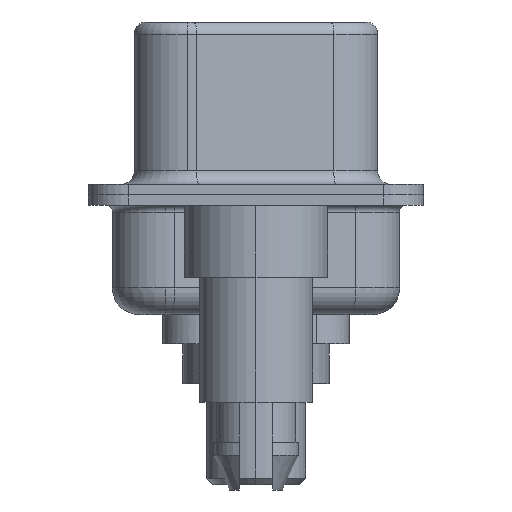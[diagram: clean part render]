
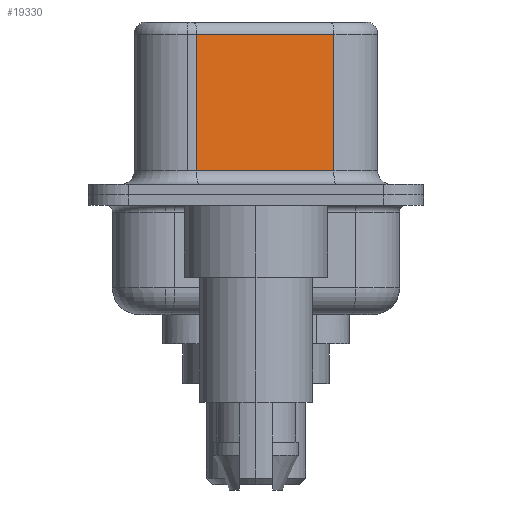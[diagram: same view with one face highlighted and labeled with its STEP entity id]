
A CAD part, left-side view. The second image highlights one B-rep face of the part: STEP entity #19330.
In plain terms, the highlighted planar face has unit normal (-0.985, -0.174, 0).
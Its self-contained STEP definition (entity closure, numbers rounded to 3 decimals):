
#17 = CARTESIAN_POINT ( 'NONE',  ( 4.585, -2.927, 6.52 ) ) ;
#502 = ORIENTED_EDGE ( 'NONE', *, *, #4506, .T. ) ;
#1041 = DIRECTION ( 'NONE',  ( -0.174, 0.985, 0. ) ) ;
#1089 = LINE ( 'NONE', #17, #16523 ) ;
#1209 = LINE ( 'NONE', #10187, #16655 ) ;
#1450 = DIRECTION ( 'NONE',  ( 0.174, -0.985, 0. ) ) ;
#4052 = EDGE_CURVE ( 'NONE', #6802, #17455, #1089, .T. ) ;
#4506 = EDGE_CURVE ( 'NONE', #6802, #15293, #11897, .T. ) ;
#5594 = CARTESIAN_POINT ( 'NONE',  ( 4.585, -2.927, 6.52 ) ) ;
#5728 = ORIENTED_EDGE ( 'NONE', *, *, #4052, .F. ) ;
#5755 = CARTESIAN_POINT ( 'NONE',  ( 3.675, 2.233, 6.02 ) ) ;
#6802 = VERTEX_POINT ( 'NONE', #10339 ) ;
#7949 = EDGE_CURVE ( 'NONE', #15293, #10622, #1209, .T. ) ;
#8872 = ORIENTED_EDGE ( 'NONE', *, *, #7949, .T. ) ;
#9713 = CARTESIAN_POINT ( 'NONE',  ( 3.675, 2.233, 0.9 ) ) ;
#10095 = DIRECTION ( 'NONE',  ( 0.985, 0.174, 0. ) ) ;
#10187 = CARTESIAN_POINT ( 'NONE',  ( 3.675, 2.233, 6.52 ) ) ;
#10339 = CARTESIAN_POINT ( 'NONE',  ( 4.585, -2.927, 6.02 ) ) ;
#10622 = VERTEX_POINT ( 'NONE', #9713 ) ;
#10651 = ORIENTED_EDGE ( 'NONE', *, *, #15370, .T. ) ;
#11198 = AXIS2_PLACEMENT_3D ( 'NONE', #5594, #10095, #1041 ) ;
#11897 = LINE ( 'NONE', #12663, #15821 ) ;
#11906 = CARTESIAN_POINT ( 'NONE',  ( 4.585, -2.927, 0.9 ) ) ;
#12293 = DIRECTION ( 'NONE',  ( 0., 0., -1. ) ) ;
#12663 = CARTESIAN_POINT ( 'NONE',  ( 4.585, -2.927, 6.02 ) ) ;
#13154 = VECTOR ( 'NONE', #1450, 1000. ) ;
#13705 = EDGE_LOOP ( 'NONE', ( #5728, #502, #8872, #10651 ) ) ;
#14837 = CARTESIAN_POINT ( 'NONE',  ( 4.585, -2.927, 0.9 ) ) ;
#15293 = VERTEX_POINT ( 'NONE', #5755 ) ;
#15370 = EDGE_CURVE ( 'NONE', #10622, #17455, #17102, .T. ) ;
#15821 = VECTOR ( 'NONE', #18041, 1000. ) ;
#16069 = FACE_OUTER_BOUND ( 'NONE', #13705, .T. ) ;
#16523 = VECTOR ( 'NONE', #12293, 1000. ) ;
#16655 = VECTOR ( 'NONE', #19116, 1000. ) ;
#17102 = LINE ( 'NONE', #11906, #13154 ) ;
#17455 = VERTEX_POINT ( 'NONE', #14837 ) ;
#18041 = DIRECTION ( 'NONE',  ( -0.174, 0.985, 0. ) ) ;
#18967 = PLANE ( 'NONE',  #11198 ) ;
#19116 = DIRECTION ( 'NONE',  ( 0., 0., -1. ) ) ;
#19330 = ADVANCED_FACE ( 'NONE', ( #16069 ), #18967, .F. ) ;
